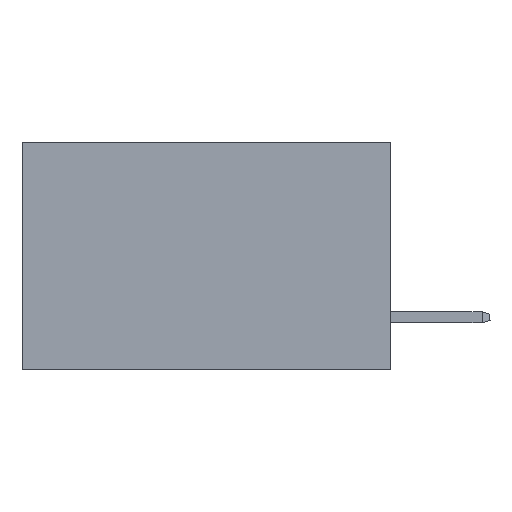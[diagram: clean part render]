
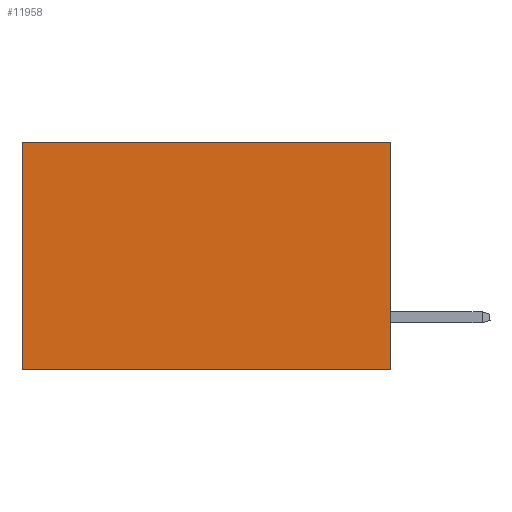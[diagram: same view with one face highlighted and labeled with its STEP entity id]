
A CAD part, left-side view. The second image highlights one B-rep face of the part: STEP entity #11958.
In plain terms, the highlighted planar face has unit normal (-1, 0, 0).
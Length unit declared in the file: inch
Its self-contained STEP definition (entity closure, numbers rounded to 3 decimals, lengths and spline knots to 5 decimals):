
#1147 = VECTOR ( 'NONE', #32082, 39.37008 ) ;
#2126 = VECTOR ( 'NONE', #16233, 39.37008 ) ;
#3242 = DIRECTION ( 'NONE',  ( 0., 0., -1. ) ) ;
#3325 = LINE ( 'NONE', #16399, #2126 ) ;
#3723 = EDGE_CURVE ( 'NONE', #44456, #45042, #25303, .T. ) ;
#5234 = CARTESIAN_POINT ( 'NONE',  ( 0.2875, 0., -0.37 ) ) ;
#7555 = CARTESIAN_POINT ( 'NONE',  ( 0.2875, 0.6, 0. ) ) ;
#8252 = LINE ( 'NONE', #38057, #10074 ) ;
#10074 = VECTOR ( 'NONE', #19380, 39.37008 ) ;
#11287 = VERTEX_POINT ( 'NONE', #13765 ) ;
#11672 = EDGE_CURVE ( 'NONE', #44456, #33113, #3325, .T. ) ;
#11958 = ADVANCED_FACE ( 'NONE', ( #44221 ), #45469, .F. ) ;
#12713 = CARTESIAN_POINT ( 'NONE',  ( 0.2875, 0., 0. ) ) ;
#13067 = ORIENTED_EDGE ( 'NONE', *, *, #11672, .F. ) ;
#13765 = CARTESIAN_POINT ( 'NONE',  ( 0.2875, 0.6, -0.37 ) ) ;
#14831 = CARTESIAN_POINT ( 'NONE',  ( 0.2875, 0., -0.37 ) ) ;
#16233 = DIRECTION ( 'NONE',  ( 0., 0., -1. ) ) ;
#16399 = CARTESIAN_POINT ( 'NONE',  ( 0.2875, 0., 0. ) ) ;
#19380 = DIRECTION ( 'NONE',  ( 0., 0., -1. ) ) ;
#20163 = ORIENTED_EDGE ( 'NONE', *, *, #3723, .T. ) ;
#21967 = CARTESIAN_POINT ( 'NONE',  ( 0.2875, 0., 0. ) ) ;
#23859 = EDGE_LOOP ( 'NONE', ( #32822, #46770, #13067, #20163 ) ) ;
#25303 = LINE ( 'NONE', #12713, #1147 ) ;
#25825 = DIRECTION ( 'NONE',  ( 1., 0., 0. ) ) ;
#30756 = LINE ( 'NONE', #5234, #45796 ) ;
#31028 = AXIS2_PLACEMENT_3D ( 'NONE', #21967, #25825, #3242 ) ;
#32082 = DIRECTION ( 'NONE',  ( 0., 1., 0. ) ) ;
#32214 = DIRECTION ( 'NONE',  ( 0., 1., 0. ) ) ;
#32822 = ORIENTED_EDGE ( 'NONE', *, *, #45106, .T. ) ;
#33113 = VERTEX_POINT ( 'NONE', #14831 ) ;
#38057 = CARTESIAN_POINT ( 'NONE',  ( 0.2875, 0.6, 0. ) ) ;
#38759 = CARTESIAN_POINT ( 'NONE',  ( 0.2875, 0., 0. ) ) ;
#44221 = FACE_OUTER_BOUND ( 'NONE', #23859, .T. ) ;
#44456 = VERTEX_POINT ( 'NONE', #38759 ) ;
#45042 = VERTEX_POINT ( 'NONE', #7555 ) ;
#45106 = EDGE_CURVE ( 'NONE', #45042, #11287, #8252, .T. ) ;
#45469 = PLANE ( 'NONE',  #31028 ) ;
#45796 = VECTOR ( 'NONE', #32214, 39.37008 ) ;
#46770 = ORIENTED_EDGE ( 'NONE', *, *, #49403, .F. ) ;
#49403 = EDGE_CURVE ( 'NONE', #33113, #11287, #30756, .T. ) ;
